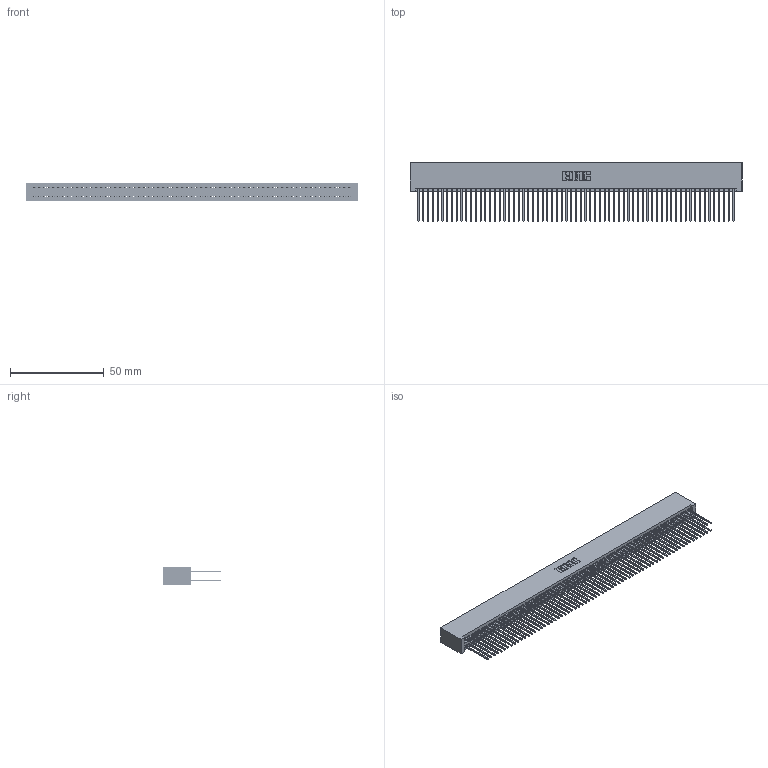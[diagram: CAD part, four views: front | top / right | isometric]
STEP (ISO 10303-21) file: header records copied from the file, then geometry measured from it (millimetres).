
FILE_DESCRIPTION (( 'STEP AP203' ), '1' );
FILE_NAME ('345-134-542-201.STEP', '2018-10-20T09:34:25', ( '' ), ( '' ), 'SwSTEP 2.0', 'SolidWorks 2016', '' );
FILE_SCHEMA (( 'CONFIG_CONTROL_DESIGN' ));
Length unit declared in the file: inch
Products named in the file (3): 345-134-542-201; 345-292-001_345-293-142; 345 Part_No Mounting Lugs
Assembly tree (135 placements, depth 2):
  345-134-542-201
    345 Part_No Mounting Lugs
    345-292-001_345-293-142  x134
Bounding box: 176.78 x 31.29 x 9.4 mm (x, y, z)
Volume: 18645.6 mm3; surface area: 31268 mm2
Topology: 135 solids, 135 shells, 6818 faces, 20283 edges, 13342 vertices
Faces by surface type: plane 4498, cylinder 2320
Entity records: 48945 total; most frequent: CARTESIAN_POINT 8180, ORIENTED_EDGE 8114, DIRECTION 7177, EDGE_CURVE 4057, VECTOR 3665, LINE 3665, VERTEX_POINT 2702, AXIS2_PLACEMENT_3D 1756
